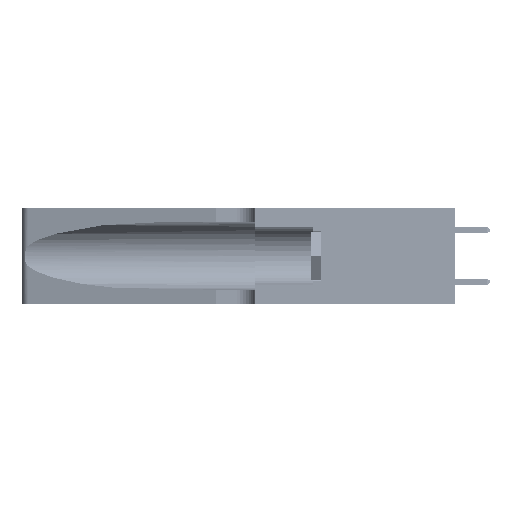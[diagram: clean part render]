
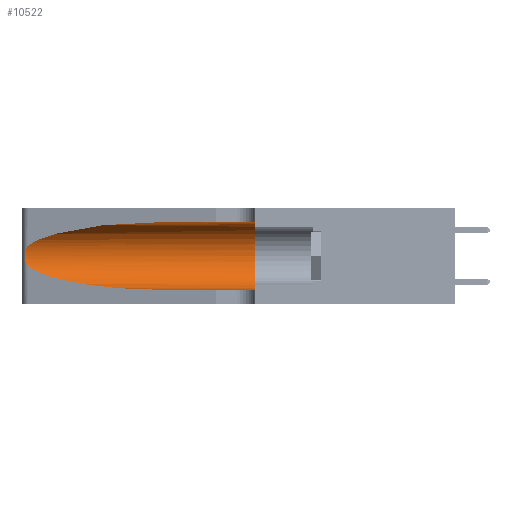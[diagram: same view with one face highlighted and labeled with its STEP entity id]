
A CAD part, left-side view. The second image highlights one B-rep face of the part: STEP entity #10522.
In plain terms, the highlighted cylindrical face has radius 3.308 mm (diameter 6.617 mm), a partial arc.
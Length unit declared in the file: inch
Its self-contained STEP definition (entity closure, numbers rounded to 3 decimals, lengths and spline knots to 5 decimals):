
#207 = CARTESIAN_POINT ( 'NONE',  ( 0.25487, 1.22718, 0.22369 ) ) ;
#231 = CARTESIAN_POINT ( 'NONE',  ( 0.1305, 1.61858, 0.05475 ) ) ;
#378 = CYLINDRICAL_SURFACE ( 'NONE', #45921, 0.13025 ) ;
#725 = DIRECTION ( 'NONE',  ( 0., -1., 0. ) ) ;
#1932 = CARTESIAN_POINT ( 'NONE',  ( 0.2373, 1.15595, 0.28018 ) ) ;
#2178 = VERTEX_POINT ( 'NONE', #44209 ) ;
#2669 = EDGE_CURVE ( 'NONE', #46520, #35884, #33172, .T. ) ;
#4184 = CARTESIAN_POINT ( 'NONE',  ( 0.25854, 1.2359, 0.20912 ) ) ;
#4213 =( BOUNDED_CURVE ( )  B_SPLINE_CURVE ( 3, ( #33171, #21483, #1932, #29390 ),
 .UNSPECIFIED., .F., .F. ) 
 B_SPLINE_CURVE_WITH_KNOTS ( ( 4, 4 ),
 ( 1.5708, 2.84003 ),
 .UNSPECIFIED. ) 
 CURVE ( )  GEOMETRIC_REPRESENTATION_ITEM ( )  RATIONAL_B_SPLINE_CURVE ( ( 1., 0.87, 0.87, 1. ) ) 
 REPRESENTATION_ITEM ( '' )  );
#4265 = EDGE_CURVE ( 'NONE', #16189, #33697, #44495, .T. ) ;
#4683 = DIRECTION ( 'NONE',  ( 0., 1., 0. ) ) ;
#8099 = CARTESIAN_POINT ( 'NONE',  ( 0.26075, 1.23896, 0.19203 ) ) ;
#8264 = VERTEX_POINT ( 'NONE', #50628 ) ;
#10522 = ADVANCED_FACE ( 'NONE', ( #42191 ), #378, .F. ) ;
#11619 = LINE ( 'NONE', #231, #43008 ) ;
#11890 = DIRECTION ( 'NONE',  ( 0., -1., 0. ) ) ;
#12022 = CARTESIAN_POINT ( 'NONE',  ( 0.26017, 1.23833, 0.17102 ) ) ;
#13312 = ORIENTED_EDGE ( 'NONE', *, *, #20293, .T. ) ;
#15249 = EDGE_CURVE ( 'NONE', #2178, #35884, #11619, .T. ) ;
#15802 = ORIENTED_EDGE ( 'NONE', *, *, #20265, .F. ) ;
#16017 = CARTESIAN_POINT ( 'NONE',  ( 0.25789, 1.23486, 0.15765 ) ) ;
#16189 = VERTEX_POINT ( 'NONE', #32248 ) ;
#18151 = EDGE_LOOP ( 'NONE', ( #41600, #26696, #13312, #29055, #39469, #15802 ) ) ;
#19654 = CARTESIAN_POINT ( 'NONE',  ( 0.25487, 1.22718, 0.14631 ) ) ;
#19948 = CARTESIAN_POINT ( 'NONE',  ( 0.25555, 1.22993, 0.14849 ) ) ;
#20265 = EDGE_CURVE ( 'NONE', #8264, #46520, #32687, .T. ) ;
#20293 = EDGE_CURVE ( 'NONE', #33697, #2178, #49847, .T. ) ;
#20308 = DIRECTION ( 'NONE',  ( 0., 0., -1. ) ) ;
#21483 = CARTESIAN_POINT ( 'NONE',  ( 0.18966, 0.96281, 0.31525 ) ) ;
#22079 = AXIS2_PLACEMENT_3D ( 'NONE', #28197, #4683, #32153 ) ;
#22242 = VECTOR ( 'NONE', #11890, 39.37008 ) ;
#23609 = CARTESIAN_POINT ( 'NONE',  ( 0.1305, 1.61858, 0.31525 ) ) ;
#23779 = CARTESIAN_POINT ( 'NONE',  ( 0.1305, 0.72297, 0.05475 ) ) ;
#26696 = ORIENTED_EDGE ( 'NONE', *, *, #4265, .T. ) ;
#27694 = CARTESIAN_POINT ( 'NONE',  ( 0.25787, 1.23484, 0.2124 ) ) ;
#27712 = DIRECTION ( 'NONE',  ( 0., -1., 0. ) ) ;
#28197 = CARTESIAN_POINT ( 'NONE',  ( 0.1305, 0.35, 0.185 ) ) ;
#29055 = ORIENTED_EDGE ( 'NONE', *, *, #15249, .T. ) ;
#29390 = CARTESIAN_POINT ( 'NONE',  ( 0.25487, 1.22718, 0.22369 ) ) ;
#31630 = CARTESIAN_POINT ( 'NONE',  ( 0.26018, 1.23835, 0.19895 ) ) ;
#32153 = DIRECTION ( 'NONE',  ( 0., 0., 1. ) ) ;
#32248 = CARTESIAN_POINT ( 'NONE',  ( 0.25487, 1.22718, 0.22369 ) ) ;
#32687 = LINE ( 'NONE', #23609, #22242 ) ;
#33171 = CARTESIAN_POINT ( 'NONE',  ( 0.1305, 0.72297, 0.31525 ) ) ;
#33172 = CIRCLE ( 'NONE', #22079, 0.13025 ) ;
#33697 = VERTEX_POINT ( 'NONE', #40246 ) ;
#35352 = CARTESIAN_POINT ( 'NONE',  ( 0.1305, 0.35, 0.05475 ) ) ;
#35407 = CARTESIAN_POINT ( 'NONE',  ( 0.25639, 1.23184, 0.21858 ) ) ;
#35582 = CARTESIAN_POINT ( 'NONE',  ( 0.26075, 1.23896, 0.178 ) ) ;
#35884 = VERTEX_POINT ( 'NONE', #35352 ) ;
#39364 = CARTESIAN_POINT ( 'NONE',  ( 0.25555, 1.22994, 0.2215 ) ) ;
#39469 = ORIENTED_EDGE ( 'NONE', *, *, #2669, .F. ) ;
#39542 = CARTESIAN_POINT ( 'NONE',  ( 0.25856, 1.23593, 0.16098 ) ) ;
#40246 = CARTESIAN_POINT ( 'NONE',  ( 0.25487, 1.22718, 0.14631 ) ) ;
#41600 = ORIENTED_EDGE ( 'NONE', *, *, #46053, .T. ) ;
#42191 = FACE_OUTER_BOUND ( 'NONE', #18151, .T. ) ;
#43008 = VECTOR ( 'NONE', #27712, 39.37008 ) ;
#43361 = CARTESIAN_POINT ( 'NONE',  ( 0.2373, 1.15595, 0.08982 ) ) ;
#43496 = CARTESIAN_POINT ( 'NONE',  ( 0.25639, 1.23186, 0.15144 ) ) ;
#44209 = CARTESIAN_POINT ( 'NONE',  ( 0.1305, 0.72297, 0.05475 ) ) ;
#44495 = B_SPLINE_CURVE_WITH_KNOTS ( 'NONE', 3,
 ( #207, #39364, #35407, #27694, #4184, #31630, #8099, #35582, #12022, #39542, #16017, #43496, #19948, #47466 ),
 .UNSPECIFIED., .F., .F.,
 ( 4, 2, 2, 2, 2, 2, 4 ),
 ( 0., 0.00027, 0.00053, 0.00107, 0.0016, 0.00187, 0.00214 ),
 .UNSPECIFIED. ) ;
#45921 = AXIS2_PLACEMENT_3D ( 'NONE', #47816, #725, #20308 ) ;
#46053 = EDGE_CURVE ( 'NONE', #8264, #16189, #4213, .T. ) ;
#46520 = VERTEX_POINT ( 'NONE', #47577 ) ;
#47333 = CARTESIAN_POINT ( 'NONE',  ( 0.18966, 0.96281, 0.05475 ) ) ;
#47466 = CARTESIAN_POINT ( 'NONE',  ( 0.25487, 1.22718, 0.14631 ) ) ;
#47577 = CARTESIAN_POINT ( 'NONE',  ( 0.1305, 0.35, 0.31525 ) ) ;
#47816 = CARTESIAN_POINT ( 'NONE',  ( 0.1305, 1.61858, 0.185 ) ) ;
#49847 =( BOUNDED_CURVE ( )  B_SPLINE_CURVE ( 3, ( #19654, #43361, #47333, #23779 ),
 .UNSPECIFIED., .F., .F. ) 
 B_SPLINE_CURVE_WITH_KNOTS ( ( 4, 4 ),
 ( 3.44316, 4.71239 ),
 .UNSPECIFIED. ) 
 CURVE ( )  GEOMETRIC_REPRESENTATION_ITEM ( )  RATIONAL_B_SPLINE_CURVE ( ( 1., 0.87, 0.87, 1. ) ) 
 REPRESENTATION_ITEM ( '' )  );
#50628 = CARTESIAN_POINT ( 'NONE',  ( 0.1305, 0.72297, 0.31525 ) ) ;
